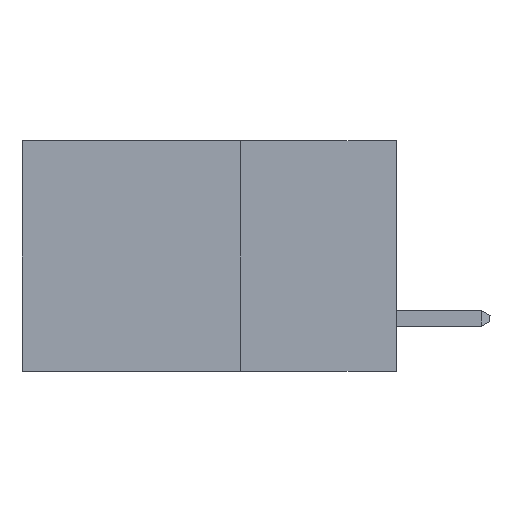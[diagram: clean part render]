
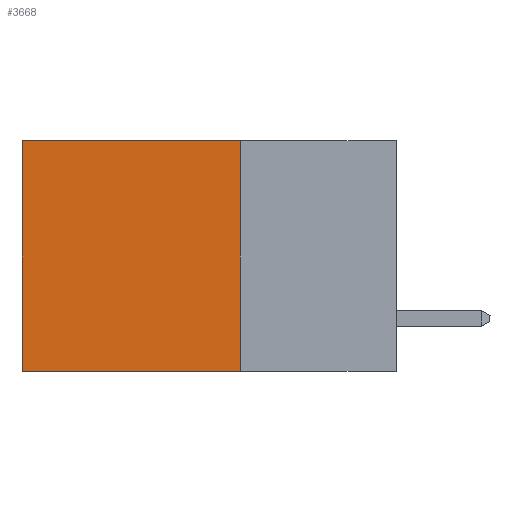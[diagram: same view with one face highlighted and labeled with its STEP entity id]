
A CAD part, left-side view. The second image highlights one B-rep face of the part: STEP entity #3668.
In plain terms, the highlighted planar face has unit normal (-1, 0, 0).
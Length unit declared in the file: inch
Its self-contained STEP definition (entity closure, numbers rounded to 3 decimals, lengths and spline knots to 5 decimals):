
#167 = LINE ( 'NONE', #7041, #7361 ) ;
#1594 = EDGE_LOOP ( 'NONE', ( #8142, #2407, #13441, #4145 ) ) ;
#2407 = ORIENTED_EDGE ( 'NONE', *, *, #3312, .F. ) ;
#3162 = CARTESIAN_POINT ( 'NONE',  ( 0.2615, 0.25, -0.37 ) ) ;
#3312 = EDGE_CURVE ( 'NONE', #3983, #11142, #14850, .T. ) ;
#3668 = ADVANCED_FACE ( 'NONE', ( #11957 ), #5936, .F. ) ;
#3983 = VERTEX_POINT ( 'NONE', #6000 ) ;
#4145 = ORIENTED_EDGE ( 'NONE', *, *, #13006, .T. ) ;
#4416 = VECTOR ( 'NONE', #14882, 39.37008 ) ;
#4744 = CARTESIAN_POINT ( 'NONE',  ( 0.2615, 0.6, 0. ) ) ;
#5936 = PLANE ( 'NONE',  #13864 ) ;
#6000 = CARTESIAN_POINT ( 'NONE',  ( 0.2615, 0.25, -0.37 ) ) ;
#6437 = VECTOR ( 'NONE', #10386, 39.37008 ) ;
#6663 = VERTEX_POINT ( 'NONE', #14235 ) ;
#7041 = CARTESIAN_POINT ( 'NONE',  ( 0.2615, 0.6, -0.37 ) ) ;
#7066 = EDGE_CURVE ( 'NONE', #6663, #3983, #16269, .T. ) ;
#7276 = VECTOR ( 'NONE', #15151, 39.37008 ) ;
#7347 = DIRECTION ( 'NONE',  ( 0., 0., -1. ) ) ;
#7361 = VECTOR ( 'NONE', #8299, 39.37008 ) ;
#8142 = ORIENTED_EDGE ( 'NONE', *, *, #9272, .T. ) ;
#8299 = DIRECTION ( 'NONE',  ( 0., 0., -1. ) ) ;
#9272 = EDGE_CURVE ( 'NONE', #12835, #11142, #167, .T. ) ;
#10386 = DIRECTION ( 'NONE',  ( 0., 0., -1. ) ) ;
#10425 = CARTESIAN_POINT ( 'NONE',  ( 0.2615, 0.25, -0.37 ) ) ;
#10552 = LINE ( 'NONE', #15031, #7276 ) ;
#11142 = VERTEX_POINT ( 'NONE', #15208 ) ;
#11957 = FACE_OUTER_BOUND ( 'NONE', #1594, .T. ) ;
#11962 = DIRECTION ( 'NONE',  ( 1., 0., 0. ) ) ;
#12835 = VERTEX_POINT ( 'NONE', #4744 ) ;
#13006 = EDGE_CURVE ( 'NONE', #6663, #12835, #10552, .T. ) ;
#13441 = ORIENTED_EDGE ( 'NONE', *, *, #7066, .F. ) ;
#13864 = AXIS2_PLACEMENT_3D ( 'NONE', #3162, #11962, #7347 ) ;
#14235 = CARTESIAN_POINT ( 'NONE',  ( 0.2615, 0.25, 0. ) ) ;
#14850 = LINE ( 'NONE', #15061, #4416 ) ;
#14882 = DIRECTION ( 'NONE',  ( 0., 1., 0. ) ) ;
#15031 = CARTESIAN_POINT ( 'NONE',  ( 0.2615, 0.25, 0. ) ) ;
#15061 = CARTESIAN_POINT ( 'NONE',  ( 0.2615, 0.25, -0.37 ) ) ;
#15151 = DIRECTION ( 'NONE',  ( 0., 1., 0. ) ) ;
#15208 = CARTESIAN_POINT ( 'NONE',  ( 0.2615, 0.6, -0.37 ) ) ;
#16269 = LINE ( 'NONE', #10425, #6437 ) ;
